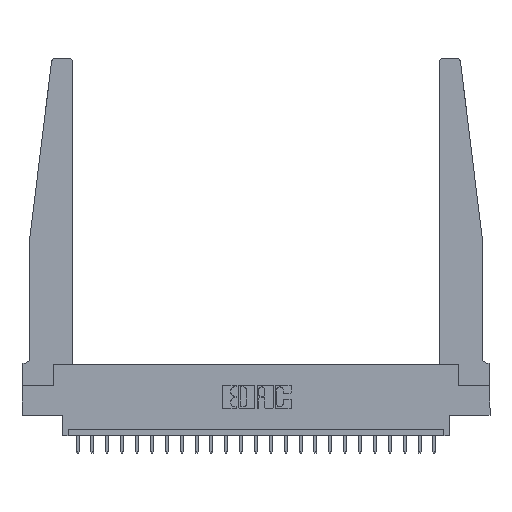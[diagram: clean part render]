
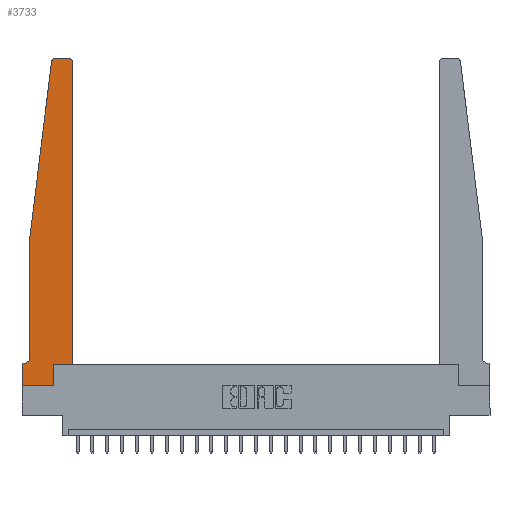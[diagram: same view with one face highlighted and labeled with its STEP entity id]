
A CAD part, top view. The second image highlights one B-rep face of the part: STEP entity #3733.
In plain terms, the highlighted planar face has unit normal (0, 0, 1).
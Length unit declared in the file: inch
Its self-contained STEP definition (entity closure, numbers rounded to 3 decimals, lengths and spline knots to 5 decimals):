
#480 = AXIS2_PLACEMENT_3D ( 'NONE', #5374, #17665, #10704 ) ;
#564 = CARTESIAN_POINT ( 'NONE',  ( 0.065, 0.2375, 0.37 ) ) ;
#608 = CARTESIAN_POINT ( 'NONE',  ( 0.2605, 0., 0.37 ) ) ;
#1225 = VECTOR ( 'NONE', #14232, 39.37008 ) ;
#1404 = DIRECTION ( 'NONE',  ( -1., 0., 0. ) ) ;
#1524 = CARTESIAN_POINT ( 'NONE',  ( 0.015, 0.1875, 0.37 ) ) ;
#1736 = DIRECTION ( 'NONE',  ( -0.122, -0.992, 0. ) ) ;
#1858 = VECTOR ( 'NONE', #2221, 39.37008 ) ;
#1950 = CARTESIAN_POINT ( 'NONE',  ( 0.25, 2.75, 0.37 ) ) ;
#1994 = LINE ( 'NONE', #2545, #6402 ) ;
#2221 = DIRECTION ( 'NONE',  ( 0., -1., 0. ) ) ;
#2545 = CARTESIAN_POINT ( 'NONE',  ( 0.065, 1.25, 0.37 ) ) ;
#2650 = ORIENTED_EDGE ( 'NONE', *, *, #11016, .T. ) ;
#3087 = ORIENTED_EDGE ( 'NONE', *, *, #18997, .T. ) ;
#3394 = CARTESIAN_POINT ( 'NONE',  ( 0., 0., 0.37 ) ) ;
#3614 = ORIENTED_EDGE ( 'NONE', *, *, #12201, .T. ) ;
#3715 = CIRCLE ( 'NONE', #14319, 0.05 ) ;
#3733 = ADVANCED_FACE ( 'NONE', ( #14977 ), #9838, .T. ) ;
#3848 = CARTESIAN_POINT ( 'NONE',  ( 0.425, 2.72, 0.37 ) ) ;
#3865 = VERTEX_POINT ( 'NONE', #1524 ) ;
#4323 = CARTESIAN_POINT ( 'NONE',  ( 0.015, 0.2375, 0.37 ) ) ;
#4520 = ORIENTED_EDGE ( 'NONE', *, *, #10568, .T. ) ;
#5361 = VECTOR ( 'NONE', #10096, 39.37008 ) ;
#5374 = CARTESIAN_POINT ( 'NONE',  ( 0.395, 2.72, 0.37 ) ) ;
#5761 = CARTESIAN_POINT ( 'NONE',  ( 0.27653, 2.75, 0.37 ) ) ;
#5924 = LINE ( 'NONE', #1950, #1225 ) ;
#5982 = VECTOR ( 'NONE', #9132, 39.37008 ) ;
#6271 = CARTESIAN_POINT ( 'NONE',  ( 0.27653, 2.72, 0.37 ) ) ;
#6320 = DIRECTION ( 'NONE',  ( 1., 0., 0. ) ) ;
#6402 = VECTOR ( 'NONE', #1736, 39.37008 ) ;
#7057 = LINE ( 'NONE', #3394, #8973 ) ;
#7371 = LINE ( 'NONE', #12667, #1858 ) ;
#7412 = CIRCLE ( 'NONE', #480, 0.03 ) ;
#7970 = ORIENTED_EDGE ( 'NONE', *, *, #14989, .T. ) ;
#8346 = VECTOR ( 'NONE', #13817, 39.37008 ) ;
#8683 = LINE ( 'NONE', #17073, #13363 ) ;
#8973 = VECTOR ( 'NONE', #20980, 39.37008 ) ;
#9132 = DIRECTION ( 'NONE',  ( 1., 0., 0. ) ) ;
#9331 = VERTEX_POINT ( 'NONE', #20478 ) ;
#9415 = DIRECTION ( 'NONE',  ( -1., 0., 0. ) ) ;
#9838 = PLANE ( 'NONE',  #21502 ) ;
#9860 = DIRECTION ( 'NONE',  ( 0., 0., 1. ) ) ;
#10096 = DIRECTION ( 'NONE',  ( 0., 1., 0. ) ) ;
#10388 = VERTEX_POINT ( 'NONE', #11978 ) ;
#10568 = EDGE_CURVE ( 'NONE', #15740, #19960, #21916, .T. ) ;
#10632 = VERTEX_POINT ( 'NONE', #19766 ) ;
#10684 = VECTOR ( 'NONE', #14064, 39.37008 ) ;
#10704 = DIRECTION ( 'NONE',  ( 1., 0., 0. ) ) ;
#10769 = VERTEX_POINT ( 'NONE', #564 ) ;
#11016 = EDGE_CURVE ( 'NONE', #19750, #10388, #7057, .T. ) ;
#11038 = ORIENTED_EDGE ( 'NONE', *, *, #20989, .T. ) ;
#11154 = CIRCLE ( 'NONE', #16446, 0.03 ) ;
#11252 = VERTEX_POINT ( 'NONE', #13580 ) ;
#11763 = DIRECTION ( 'NONE',  ( 0., 0., 1. ) ) ;
#11978 = CARTESIAN_POINT ( 'NONE',  ( 0., 0., 0.37 ) ) ;
#12201 = EDGE_CURVE ( 'NONE', #9331, #13541, #5924, .T. ) ;
#12383 = CARTESIAN_POINT ( 'NONE',  ( 0.425, 0.18, 0.37 ) ) ;
#12478 = EDGE_CURVE ( 'NONE', #13541, #10632, #11154, .T. ) ;
#12667 = CARTESIAN_POINT ( 'NONE',  ( 0.065, 1.25, 0.37 ) ) ;
#12857 = LINE ( 'NONE', #14263, #5982 ) ;
#13045 = ORIENTED_EDGE ( 'NONE', *, *, #17146, .T. ) ;
#13326 = ORIENTED_EDGE ( 'NONE', *, *, #21849, .T. ) ;
#13363 = VECTOR ( 'NONE', #1404, 39.37008 ) ;
#13541 = VERTEX_POINT ( 'NONE', #5761 ) ;
#13567 = VERTEX_POINT ( 'NONE', #20347 ) ;
#13580 = CARTESIAN_POINT ( 'NONE',  ( 0.2605, 0.18, 0.37 ) ) ;
#13584 = EDGE_CURVE ( 'NONE', #10632, #13567, #1994, .T. ) ;
#13763 = ORIENTED_EDGE ( 'NONE', *, *, #13584, .T. ) ;
#13817 = DIRECTION ( 'NONE',  ( 1., 0., 0. ) ) ;
#14064 = DIRECTION ( 'NONE',  ( 0., 1., 0. ) ) ;
#14232 = DIRECTION ( 'NONE',  ( -1., 0., 0. ) ) ;
#14263 = CARTESIAN_POINT ( 'NONE',  ( 0.425, 0.18, 0.37 ) ) ;
#14319 = AXIS2_PLACEMENT_3D ( 'NONE', #4323, #21836, #9415 ) ;
#14743 = CARTESIAN_POINT ( 'NONE',  ( 0., 0., 0.37 ) ) ;
#14919 = CARTESIAN_POINT ( 'NONE',  ( 0., 0.1875, 0.37 ) ) ;
#14921 = LINE ( 'NONE', #14743, #8346 ) ;
#14977 = FACE_OUTER_BOUND ( 'NONE', #17991, .T. ) ;
#14989 = EDGE_CURVE ( 'NONE', #10388, #18958, #14921, .T. ) ;
#15740 = VERTEX_POINT ( 'NONE', #12383 ) ;
#16446 = AXIS2_PLACEMENT_3D ( 'NONE', #6271, #9860, #22053 ) ;
#16906 = CARTESIAN_POINT ( 'NONE',  ( 0., 0.1875, 0.37 ) ) ;
#17073 = CARTESIAN_POINT ( 'NONE',  ( 0.065, 0.1875, 0.37 ) ) ;
#17146 = EDGE_CURVE ( 'NONE', #19960, #9331, #7412, .T. ) ;
#17437 = CARTESIAN_POINT ( 'NONE',  ( 0.425, 0.18, 0.37 ) ) ;
#17665 = DIRECTION ( 'NONE',  ( 0., 0., 1. ) ) ;
#17991 = EDGE_LOOP ( 'NONE', ( #3614, #19731, #13763, #3087, #18162, #18061, #2650, #7970, #13326, #11038, #4520, #13045 ) ) ;
#18061 = ORIENTED_EDGE ( 'NONE', *, *, #21882, .T. ) ;
#18162 = ORIENTED_EDGE ( 'NONE', *, *, #21754, .T. ) ;
#18958 = VERTEX_POINT ( 'NONE', #608 ) ;
#18997 = EDGE_CURVE ( 'NONE', #13567, #10769, #7371, .T. ) ;
#19731 = ORIENTED_EDGE ( 'NONE', *, *, #12478, .T. ) ;
#19750 = VERTEX_POINT ( 'NONE', #14919 ) ;
#19766 = CARTESIAN_POINT ( 'NONE',  ( 0.24675, 2.72367, 0.37 ) ) ;
#19960 = VERTEX_POINT ( 'NONE', #3848 ) ;
#20347 = CARTESIAN_POINT ( 'NONE',  ( 0.065, 1.25, 0.37 ) ) ;
#20478 = CARTESIAN_POINT ( 'NONE',  ( 0.395, 2.75, 0.37 ) ) ;
#20604 = CARTESIAN_POINT ( 'NONE',  ( 0.2605, 0.18, 0.37 ) ) ;
#20980 = DIRECTION ( 'NONE',  ( 0., -1., 0. ) ) ;
#20989 = EDGE_CURVE ( 'NONE', #11252, #15740, #12857, .T. ) ;
#21502 = AXIS2_PLACEMENT_3D ( 'NONE', #16906, #11763, #6320 ) ;
#21598 = LINE ( 'NONE', #20604, #5361 ) ;
#21754 = EDGE_CURVE ( 'NONE', #10769, #3865, #3715, .T. ) ;
#21836 = DIRECTION ( 'NONE',  ( 0., 0., -1. ) ) ;
#21849 = EDGE_CURVE ( 'NONE', #18958, #11252, #21598, .T. ) ;
#21882 = EDGE_CURVE ( 'NONE', #3865, #19750, #8683, .T. ) ;
#21916 = LINE ( 'NONE', #17437, #10684 ) ;
#22053 = DIRECTION ( 'NONE',  ( 1., 0., 0. ) ) ;
